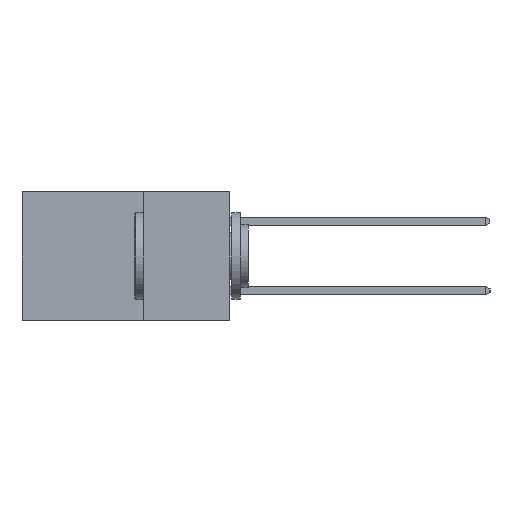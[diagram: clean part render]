
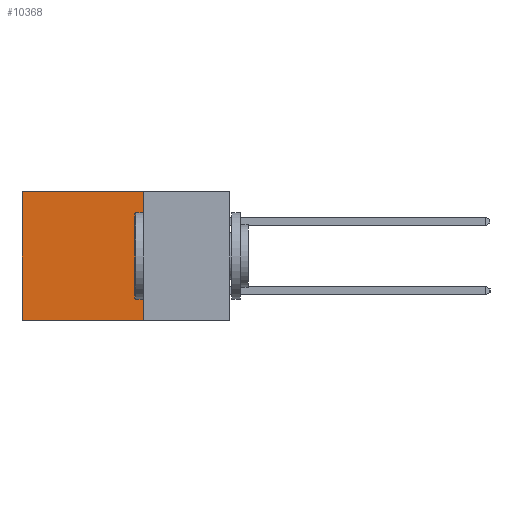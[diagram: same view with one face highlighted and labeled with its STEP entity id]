
A CAD part, left-side view. The second image highlights one B-rep face of the part: STEP entity #10368.
In plain terms, the highlighted planar face has unit normal (-1, 0, 0).
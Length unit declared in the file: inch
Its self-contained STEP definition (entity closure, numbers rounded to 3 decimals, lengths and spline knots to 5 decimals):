
#665 = CARTESIAN_POINT ( 'NONE',  ( 0.2615, 0.25, -0.37 ) ) ;
#1057 = VECTOR ( 'NONE', #5023, 39.37008 ) ;
#1265 = FACE_OUTER_BOUND ( 'NONE', #3719, .T. ) ;
#1768 = DIRECTION ( 'NONE',  ( 1., 0., 0. ) ) ;
#2118 = EDGE_CURVE ( 'NONE', #13130, #23124, #18395, .T. ) ;
#2397 = ORIENTED_EDGE ( 'NONE', *, *, #13789, .T. ) ;
#3719 = EDGE_LOOP ( 'NONE', ( #2397, #7549, #5897, #16207 ) ) ;
#3766 = AXIS2_PLACEMENT_3D ( 'NONE', #13164, #1768, #15098 ) ;
#4686 = VECTOR ( 'NONE', #11746, 39.37008 ) ;
#5023 = DIRECTION ( 'NONE',  ( 0., 0., -1. ) ) ;
#5236 = CARTESIAN_POINT ( 'NONE',  ( 0.2615, 0.25, 0. ) ) ;
#5253 = CARTESIAN_POINT ( 'NONE',  ( 0.2615, 0.6, -0.37 ) ) ;
#5897 = ORIENTED_EDGE ( 'NONE', *, *, #14037, .F. ) ;
#6073 = VECTOR ( 'NONE', #17701, 39.37008 ) ;
#6248 = VERTEX_POINT ( 'NONE', #20920 ) ;
#6672 = LINE ( 'NONE', #15807, #6073 ) ;
#6930 = CARTESIAN_POINT ( 'NONE',  ( 0.2615, 0.25, -0.37 ) ) ;
#7549 = ORIENTED_EDGE ( 'NONE', *, *, #2118, .F. ) ;
#9830 = CARTESIAN_POINT ( 'NONE',  ( 0.2615, 0.25, 0. ) ) ;
#10368 = ADVANCED_FACE ( 'NONE', ( #1265 ), #24525, .F. ) ;
#11166 = LINE ( 'NONE', #6930, #1057 ) ;
#11746 = DIRECTION ( 'NONE',  ( 0., 1., 0. ) ) ;
#13130 = VERTEX_POINT ( 'NONE', #665 ) ;
#13164 = CARTESIAN_POINT ( 'NONE',  ( 0.2615, 0.25, -0.37 ) ) ;
#13789 = EDGE_CURVE ( 'NONE', #6248, #23124, #6672, .T. ) ;
#14037 = EDGE_CURVE ( 'NONE', #18541, #13130, #11166, .T. ) ;
#15098 = DIRECTION ( 'NONE',  ( 0., 0., -1. ) ) ;
#15807 = CARTESIAN_POINT ( 'NONE',  ( 0.2615, 0.6, -0.37 ) ) ;
#16207 = ORIENTED_EDGE ( 'NONE', *, *, #18095, .T. ) ;
#17701 = DIRECTION ( 'NONE',  ( 0., 0., -1. ) ) ;
#18095 = EDGE_CURVE ( 'NONE', #18541, #6248, #19904, .T. ) ;
#18395 = LINE ( 'NONE', #22068, #22861 ) ;
#18541 = VERTEX_POINT ( 'NONE', #5236 ) ;
#19904 = LINE ( 'NONE', #9830, #4686 ) ;
#20920 = CARTESIAN_POINT ( 'NONE',  ( 0.2615, 0.6, 0. ) ) ;
#21769 = DIRECTION ( 'NONE',  ( 0., 1., 0. ) ) ;
#22068 = CARTESIAN_POINT ( 'NONE',  ( 0.2615, 0.25, -0.37 ) ) ;
#22861 = VECTOR ( 'NONE', #21769, 39.37008 ) ;
#23124 = VERTEX_POINT ( 'NONE', #5253 ) ;
#24525 = PLANE ( 'NONE',  #3766 ) ;
